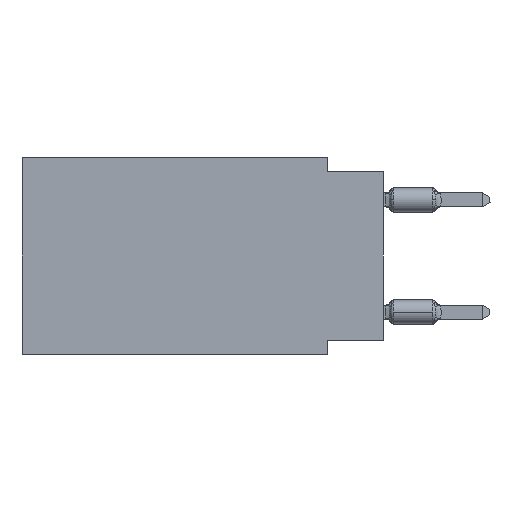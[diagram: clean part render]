
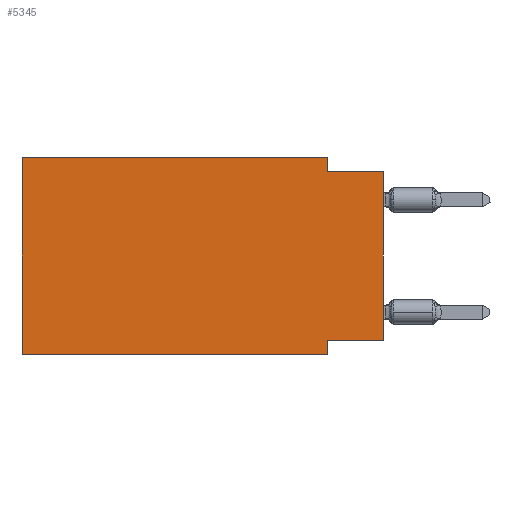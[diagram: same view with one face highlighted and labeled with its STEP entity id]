
A CAD part, left-side view. The second image highlights one B-rep face of the part: STEP entity #5345.
In plain terms, the highlighted planar face has unit normal (-1, 0, 0).
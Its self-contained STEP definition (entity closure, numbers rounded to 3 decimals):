
#248 = ORIENTED_EDGE ( 'NONE', *, *, #7531, .F. ) ;
#257 = DIRECTION ( 'NONE',  ( 0., 1., 0. ) ) ;
#425 = VERTEX_POINT ( 'NONE', #4152 ) ;
#685 = CARTESIAN_POINT ( 'NONE',  ( 0., 16.383, -8.89 ) ) ;
#1300 = CARTESIAN_POINT ( 'NONE',  ( 0., 2.54, -0.635 ) ) ;
#1549 = ORIENTED_EDGE ( 'NONE', *, *, #3981, .T. ) ;
#3004 = VERTEX_POINT ( 'NONE', #17233 ) ;
#3084 = CARTESIAN_POINT ( 'NONE',  ( 0., 2.54, -8.89 ) ) ;
#3308 = CARTESIAN_POINT ( 'NONE',  ( 0., 0., 0. ) ) ;
#3398 = EDGE_CURVE ( 'NONE', #6471, #13783, #22998, .T. ) ;
#3540 = VECTOR ( 'NONE', #10480, 1000. ) ;
#3981 = EDGE_CURVE ( 'NONE', #6471, #3004, #18044, .T. ) ;
#4152 = CARTESIAN_POINT ( 'NONE',  ( 0., 0., -8.255 ) ) ;
#4166 = FACE_OUTER_BOUND ( 'NONE', #19583, .T. ) ;
#4277 = VECTOR ( 'NONE', #5526, 1000. ) ;
#4833 = ORIENTED_EDGE ( 'NONE', *, *, #11288, .F. ) ;
#4866 = CARTESIAN_POINT ( 'NONE',  ( 0., 0., -0.635 ) ) ;
#4901 = CARTESIAN_POINT ( 'NONE',  ( 0., 16.383, 0. ) ) ;
#5345 = ADVANCED_FACE ( 'NONE', ( #4166 ), #13278, .F. ) ;
#5526 = DIRECTION ( 'NONE',  ( 0., 0., 1. ) ) ;
#6174 = VECTOR ( 'NONE', #19088, 1000. ) ;
#6471 = VERTEX_POINT ( 'NONE', #685 ) ;
#6545 = LINE ( 'NONE', #4901, #19686 ) ;
#6938 = DIRECTION ( 'NONE',  ( 0., 0., -1. ) ) ;
#7106 = ORIENTED_EDGE ( 'NONE', *, *, #18895, .T. ) ;
#7531 = EDGE_CURVE ( 'NONE', #12005, #3004, #21191, .T. ) ;
#7799 = CARTESIAN_POINT ( 'NONE',  ( 0., 0., -0.635 ) ) ;
#9382 = VECTOR ( 'NONE', #6938, 1000. ) ;
#9789 = AXIS2_PLACEMENT_3D ( 'NONE', #18403, #15248, #20392 ) ;
#10014 = CARTESIAN_POINT ( 'NONE',  ( 0., 2.54, 0. ) ) ;
#10480 = DIRECTION ( 'NONE',  ( 0., -1., 0. ) ) ;
#10541 = ORIENTED_EDGE ( 'NONE', *, *, #16389, .F. ) ;
#10860 = CARTESIAN_POINT ( 'NONE',  ( 0., 2.54, -8.255 ) ) ;
#11288 = EDGE_CURVE ( 'NONE', #18537, #16240, #19340, .T. ) ;
#11622 = EDGE_CURVE ( 'NONE', #425, #12005, #18712, .T. ) ;
#11934 = EDGE_CURVE ( 'NONE', #13783, #13222, #6545, .T. ) ;
#12005 = VERTEX_POINT ( 'NONE', #10860 ) ;
#12206 = VECTOR ( 'NONE', #257, 1000. ) ;
#12550 = LINE ( 'NONE', #3308, #4277 ) ;
#12877 = ORIENTED_EDGE ( 'NONE', *, *, #11934, .F. ) ;
#13222 = VERTEX_POINT ( 'NONE', #17414 ) ;
#13278 = PLANE ( 'NONE',  #9789 ) ;
#13783 = VERTEX_POINT ( 'NONE', #20994 ) ;
#14012 = DIRECTION ( 'NONE',  ( 0., 0., 1. ) ) ;
#14289 = CARTESIAN_POINT ( 'NONE',  ( 0., 0., -8.255 ) ) ;
#15248 = DIRECTION ( 'NONE',  ( 1., 0., 0. ) ) ;
#15416 = VECTOR ( 'NONE', #17823, 1000. ) ;
#16240 = VERTEX_POINT ( 'NONE', #7799 ) ;
#16389 = EDGE_CURVE ( 'NONE', #13222, #18537, #17127, .T. ) ;
#16872 = ORIENTED_EDGE ( 'NONE', *, *, #11622, .F. ) ;
#17127 = LINE ( 'NONE', #10014, #6174 ) ;
#17233 = CARTESIAN_POINT ( 'NONE',  ( 0., 2.54, -8.89 ) ) ;
#17252 = VECTOR ( 'NONE', #14012, 1000. ) ;
#17414 = CARTESIAN_POINT ( 'NONE',  ( 0., 2.54, 0. ) ) ;
#17698 = CARTESIAN_POINT ( 'NONE',  ( 0., 16.383, -8.89 ) ) ;
#17823 = DIRECTION ( 'NONE',  ( 0., -1., 0. ) ) ;
#18044 = LINE ( 'NONE', #17698, #15416 ) ;
#18403 = CARTESIAN_POINT ( 'NONE',  ( 0., 16.383, 0. ) ) ;
#18537 = VERTEX_POINT ( 'NONE', #1300 ) ;
#18712 = LINE ( 'NONE', #14289, #12206 ) ;
#18895 = EDGE_CURVE ( 'NONE', #425, #16240, #12550, .T. ) ;
#19088 = DIRECTION ( 'NONE',  ( 0., 0., -1. ) ) ;
#19137 = DIRECTION ( 'NONE',  ( 0., -1., 0. ) ) ;
#19340 = LINE ( 'NONE', #4866, #3540 ) ;
#19583 = EDGE_LOOP ( 'NONE', ( #7106, #4833, #10541, #12877, #20034, #1549, #248, #16872 ) ) ;
#19686 = VECTOR ( 'NONE', #19137, 1000. ) ;
#20034 = ORIENTED_EDGE ( 'NONE', *, *, #3398, .F. ) ;
#20392 = DIRECTION ( 'NONE',  ( 0., 0., -1. ) ) ;
#20994 = CARTESIAN_POINT ( 'NONE',  ( 0., 16.383, 0. ) ) ;
#21191 = LINE ( 'NONE', #3084, #9382 ) ;
#22865 = CARTESIAN_POINT ( 'NONE',  ( 0., 16.383, 0. ) ) ;
#22998 = LINE ( 'NONE', #22865, #17252 ) ;
